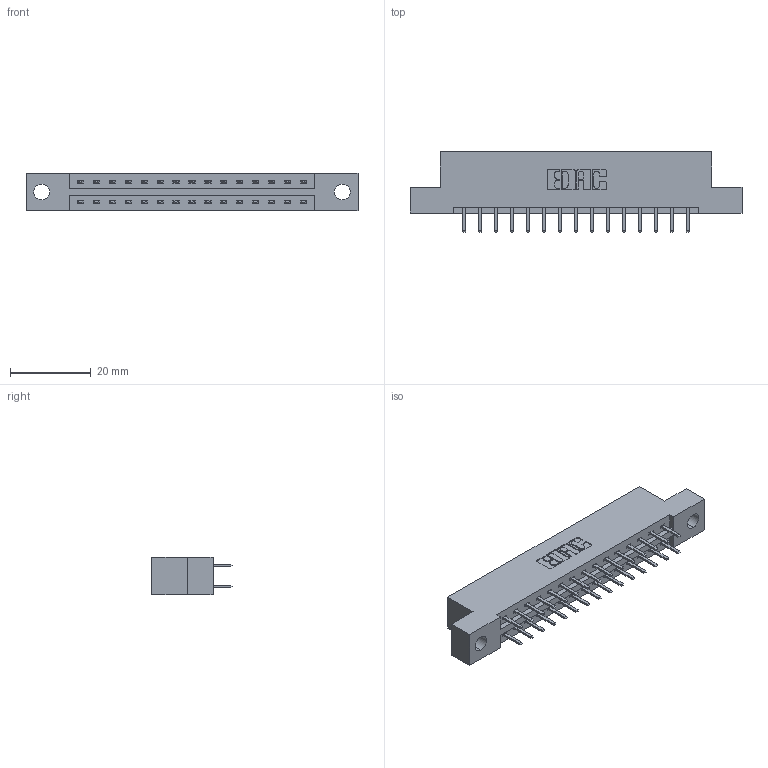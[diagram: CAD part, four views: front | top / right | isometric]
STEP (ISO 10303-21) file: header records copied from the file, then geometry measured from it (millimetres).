
FILE_DESCRIPTION (( 'STEP AP203' ), '1' );
FILE_NAME ('337-030-520-204.STEP', '2018-08-07T00:01:20', ( '' ), ( '' ), 'SwSTEP 2.0', 'SolidWorks 2016', '' );
FILE_SCHEMA (( 'CONFIG_CONTROL_DESIGN' ));
Length unit declared in the file: inch
Products named in the file (3): 337 Part_Flush Mounting Lugs - 0.156 Dia-TH; 345-292-001_345-293-120; 337-030-520-204
Assembly tree (31 placements, depth 2):
  337-030-520-204
    337 Part_Flush Mounting Lugs - 0.156 Dia-TH
    345-292-001_345-293-120  x30
Bounding box: 82.45 x 20.02 x 9.4 mm (x, y, z)
Volume: 8228.6 mm3; surface area: 8800 mm2
Topology: 31 solids, 31 shells, 1854 faces, 5381 edges, 3506 vertices
Faces by surface type: plane 1270, cylinder 584
Entity records: 15239 total; most frequent: CARTESIAN_POINT 2602, ORIENTED_EDGE 2526, DIRECTION 2251, EDGE_CURVE 1263, LINE 1131, VECTOR 1131, VERTEX_POINT 838, AXIS2_PLACEMENT_3D 560
